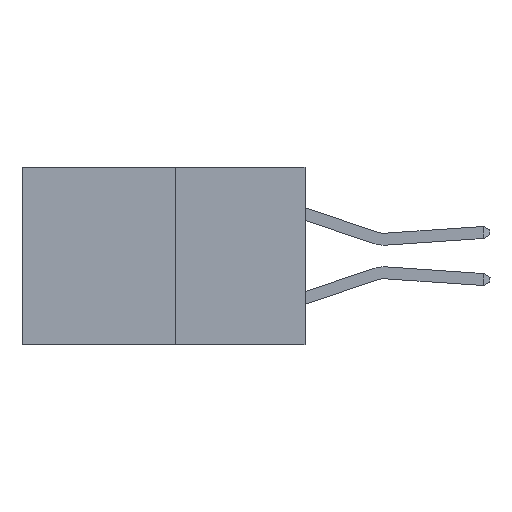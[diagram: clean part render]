
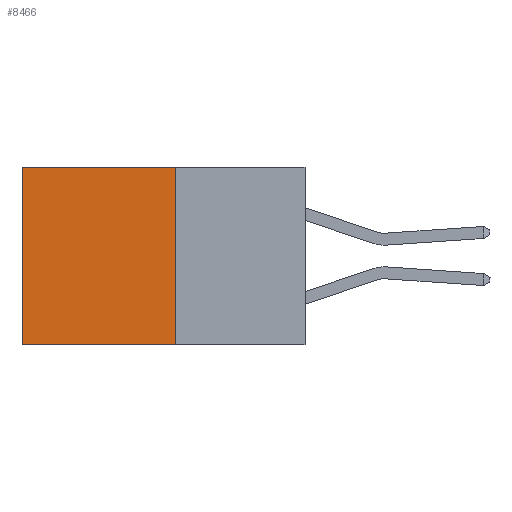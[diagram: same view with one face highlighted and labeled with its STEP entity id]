
A CAD part, left-side view. The second image highlights one B-rep face of the part: STEP entity #8466.
In plain terms, the highlighted planar face has unit normal (-1, 0, 0).
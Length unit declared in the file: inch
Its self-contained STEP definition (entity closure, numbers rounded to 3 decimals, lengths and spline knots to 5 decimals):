
#498 = EDGE_LOOP ( 'NONE', ( #3699, #28142, #12869, #13430 ) ) ;
#968 = EDGE_CURVE ( 'NONE', #11557, #9891, #12861, .T. ) ;
#1462 = LINE ( 'NONE', #21598, #19629 ) ;
#3699 = ORIENTED_EDGE ( 'NONE', *, *, #18428, .T. ) ;
#4735 = CARTESIAN_POINT ( 'NONE',  ( 0.277, 0.59, -0.37 ) ) ;
#5732 = CARTESIAN_POINT ( 'NONE',  ( 0.277, 0.27, -0.37 ) ) ;
#5838 = CARTESIAN_POINT ( 'NONE',  ( 0.277, 0.27, -0.37 ) ) ;
#6271 = VECTOR ( 'NONE', #18121, 39.37008 ) ;
#8377 = LINE ( 'NONE', #5838, #21105 ) ;
#8466 = ADVANCED_FACE ( 'NONE', ( #26188 ), #9635, .F. ) ;
#8622 = VERTEX_POINT ( 'NONE', #25792 ) ;
#9635 = PLANE ( 'NONE',  #23671 ) ;
#9891 = VERTEX_POINT ( 'NONE', #4735 ) ;
#10330 = DIRECTION ( 'NONE',  ( 0., 1., 0. ) ) ;
#11557 = VERTEX_POINT ( 'NONE', #5732 ) ;
#11878 = DIRECTION ( 'NONE',  ( 0., 0., -1. ) ) ;
#12255 = LINE ( 'NONE', #15726, #6271 ) ;
#12766 = VERTEX_POINT ( 'NONE', #18967 ) ;
#12861 = LINE ( 'NONE', #22645, #24085 ) ;
#12869 = ORIENTED_EDGE ( 'NONE', *, *, #18862, .F. ) ;
#13430 = ORIENTED_EDGE ( 'NONE', *, *, #23817, .T. ) ;
#14063 = CARTESIAN_POINT ( 'NONE',  ( 0.277, 0.27, -0.37 ) ) ;
#15726 = CARTESIAN_POINT ( 'NONE',  ( 0.277, 0.59, -0.37 ) ) ;
#18121 = DIRECTION ( 'NONE',  ( 0., 0., -1. ) ) ;
#18428 = EDGE_CURVE ( 'NONE', #12766, #9891, #12255, .T. ) ;
#18567 = DIRECTION ( 'NONE',  ( 0., 1., 0. ) ) ;
#18862 = EDGE_CURVE ( 'NONE', #8622, #11557, #8377, .T. ) ;
#18967 = CARTESIAN_POINT ( 'NONE',  ( 0.277, 0.59, 0. ) ) ;
#19417 = DIRECTION ( 'NONE',  ( 0., 0., -1. ) ) ;
#19629 = VECTOR ( 'NONE', #10330, 39.37008 ) ;
#21105 = VECTOR ( 'NONE', #19417, 39.37008 ) ;
#21598 = CARTESIAN_POINT ( 'NONE',  ( 0.277, 0.27, 0. ) ) ;
#22645 = CARTESIAN_POINT ( 'NONE',  ( 0.277, 0.27, -0.37 ) ) ;
#23671 = AXIS2_PLACEMENT_3D ( 'NONE', #14063, #25306, #11878 ) ;
#23817 = EDGE_CURVE ( 'NONE', #8622, #12766, #1462, .T. ) ;
#24085 = VECTOR ( 'NONE', #18567, 39.37008 ) ;
#25306 = DIRECTION ( 'NONE',  ( 1., 0., 0. ) ) ;
#25792 = CARTESIAN_POINT ( 'NONE',  ( 0.277, 0.27, 0. ) ) ;
#26188 = FACE_OUTER_BOUND ( 'NONE', #498, .T. ) ;
#28142 = ORIENTED_EDGE ( 'NONE', *, *, #968, .F. ) ;
